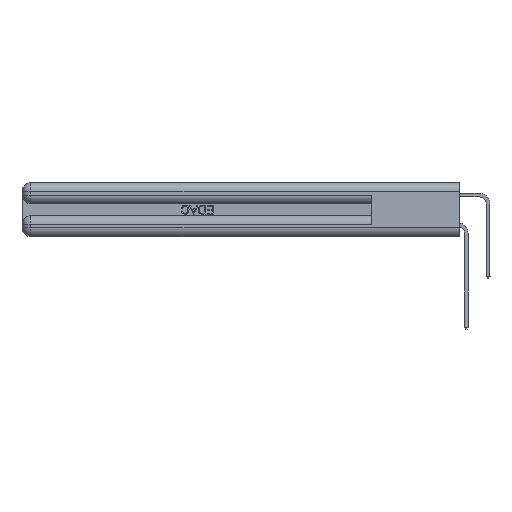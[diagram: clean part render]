
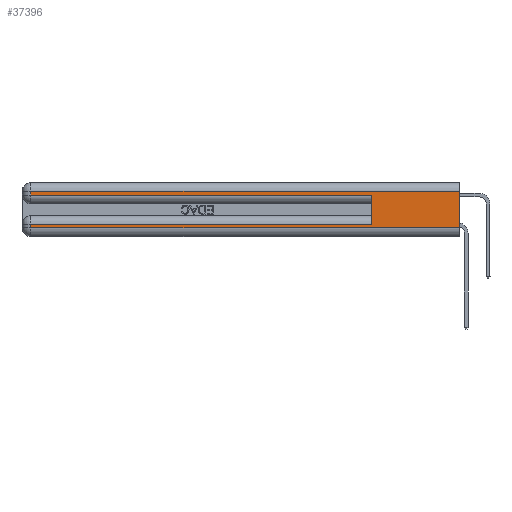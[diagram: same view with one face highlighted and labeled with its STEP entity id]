
A CAD part, left-side view. The second image highlights one B-rep face of the part: STEP entity #37396.
In plain terms, the highlighted planar face has unit normal (-1, 0, 0).
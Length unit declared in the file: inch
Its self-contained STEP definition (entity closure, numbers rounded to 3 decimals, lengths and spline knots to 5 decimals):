
#631 = ORIENTED_EDGE ( 'NONE', *, *, #49918, .T. ) ;
#2118 = VECTOR ( 'NONE', #3801, 39.37008 ) ;
#3710 = VECTOR ( 'NONE', #36872, 39.37008 ) ;
#3801 = DIRECTION ( 'NONE',  ( 0., 1., 0. ) ) ;
#4720 = AXIS2_PLACEMENT_3D ( 'NONE', #7888, #34994, #11810 ) ;
#4885 = EDGE_LOOP ( 'NONE', ( #6799, #631, #46381, #21417, #34403, #27817, #48152, #32010 ) ) ;
#5846 = CARTESIAN_POINT ( 'NONE',  ( 0., 0., 0.285 ) ) ;
#6045 = CARTESIAN_POINT ( 'NONE',  ( 0., 0.6, 0.285 ) ) ;
#6799 = ORIENTED_EDGE ( 'NONE', *, *, #39826, .F. ) ;
#7888 = CARTESIAN_POINT ( 'NONE',  ( 0., 0., 0.37 ) ) ;
#8586 = VERTEX_POINT ( 'NONE', #6045 ) ;
#8720 = CARTESIAN_POINT ( 'NONE',  ( 0., 2.94, 0.085 ) ) ;
#8737 = DIRECTION ( 'NONE',  ( 0., 0., -1. ) ) ;
#10324 = VECTOR ( 'NONE', #37346, 39.37008 ) ;
#11810 = DIRECTION ( 'NONE',  ( 0., 0., -1. ) ) ;
#13574 = CARTESIAN_POINT ( 'NONE',  ( 0., 0.6, 0.145 ) ) ;
#13713 = LINE ( 'NONE', #23196, #2118 ) ;
#14653 = VERTEX_POINT ( 'NONE', #35066 ) ;
#15236 = VERTEX_POINT ( 'NONE', #50214 ) ;
#15368 = LINE ( 'NONE', #39920, #34739 ) ;
#16518 = LINE ( 'NONE', #5846, #3710 ) ;
#16534 = CARTESIAN_POINT ( 'NONE',  ( 0., 2.94, 0.37 ) ) ;
#20644 = LINE ( 'NONE', #33439, #10324 ) ;
#20999 = CARTESIAN_POINT ( 'NONE',  ( 0., 2.94, 0.285 ) ) ;
#21417 = ORIENTED_EDGE ( 'NONE', *, *, #37201, .T. ) ;
#22734 = CARTESIAN_POINT ( 'NONE',  ( 0., 2.94, 0.31 ) ) ;
#23054 = CARTESIAN_POINT ( 'NONE',  ( 0., 0., 0.06 ) ) ;
#23059 = EDGE_CURVE ( 'NONE', #23423, #8586, #48629, .T. ) ;
#23196 = CARTESIAN_POINT ( 'NONE',  ( 0., 0., 0.31 ) ) ;
#23423 = VERTEX_POINT ( 'NONE', #50074 ) ;
#25125 = DIRECTION ( 'NONE',  ( 0., 0., 1. ) ) ;
#25429 = VERTEX_POINT ( 'NONE', #44384 ) ;
#26469 = VERTEX_POINT ( 'NONE', #8720 ) ;
#27817 = ORIENTED_EDGE ( 'NONE', *, *, #43580, .T. ) ;
#27834 = VERTEX_POINT ( 'NONE', #20999 ) ;
#29047 = VECTOR ( 'NONE', #38485, 39.37008 ) ;
#30247 = LINE ( 'NONE', #34555, #29047 ) ;
#30861 = EDGE_CURVE ( 'NONE', #25429, #15236, #43691, .T. ) ;
#32010 = ORIENTED_EDGE ( 'NONE', *, *, #30861, .T. ) ;
#33439 = CARTESIAN_POINT ( 'NONE',  ( 0., 0., 0.37 ) ) ;
#33640 = EDGE_CURVE ( 'NONE', #26469, #25429, #37393, .T. ) ;
#34403 = ORIENTED_EDGE ( 'NONE', *, *, #23059, .F. ) ;
#34555 = CARTESIAN_POINT ( 'NONE',  ( 0., 2.94, 0.37 ) ) ;
#34739 = VECTOR ( 'NONE', #47652, 39.37008 ) ;
#34821 = PLANE ( 'NONE',  #4720 ) ;
#34994 = DIRECTION ( 'NONE',  ( 1., 0., 0. ) ) ;
#35066 = CARTESIAN_POINT ( 'NONE',  ( 0., 0., 0.31 ) ) ;
#36472 = FACE_OUTER_BOUND ( 'NONE', #4885, .T. ) ;
#36872 = DIRECTION ( 'NONE',  ( 0., -1., 0. ) ) ;
#37156 = VECTOR ( 'NONE', #25125, 39.37008 ) ;
#37201 = EDGE_CURVE ( 'NONE', #27834, #8586, #16518, .T. ) ;
#37346 = DIRECTION ( 'NONE',  ( 0., 0., -1. ) ) ;
#37393 = LINE ( 'NONE', #16534, #46457 ) ;
#37396 = ADVANCED_FACE ( 'NONE', ( #36472 ), #34821, .F. ) ;
#38485 = DIRECTION ( 'NONE',  ( 0., 0., -1. ) ) ;
#39826 = EDGE_CURVE ( 'NONE', #14653, #15236, #20644, .T. ) ;
#39920 = CARTESIAN_POINT ( 'NONE',  ( 0., 0., 0.085 ) ) ;
#42472 = VERTEX_POINT ( 'NONE', #22734 ) ;
#43580 = EDGE_CURVE ( 'NONE', #23423, #26469, #15368, .T. ) ;
#43691 = LINE ( 'NONE', #23054, #46093 ) ;
#44384 = CARTESIAN_POINT ( 'NONE',  ( 0., 2.94, 0.06 ) ) ;
#46093 = VECTOR ( 'NONE', #50081, 39.37008 ) ;
#46381 = ORIENTED_EDGE ( 'NONE', *, *, #47788, .T. ) ;
#46457 = VECTOR ( 'NONE', #8737, 39.37008 ) ;
#47652 = DIRECTION ( 'NONE',  ( 0., 1., 0. ) ) ;
#47788 = EDGE_CURVE ( 'NONE', #42472, #27834, #30247, .T. ) ;
#48152 = ORIENTED_EDGE ( 'NONE', *, *, #33640, .T. ) ;
#48629 = LINE ( 'NONE', #13574, #37156 ) ;
#49918 = EDGE_CURVE ( 'NONE', #14653, #42472, #13713, .T. ) ;
#50074 = CARTESIAN_POINT ( 'NONE',  ( 0., 0.6, 0.085 ) ) ;
#50081 = DIRECTION ( 'NONE',  ( 0., -1., 0. ) ) ;
#50214 = CARTESIAN_POINT ( 'NONE',  ( 0., 0., 0.06 ) ) ;
